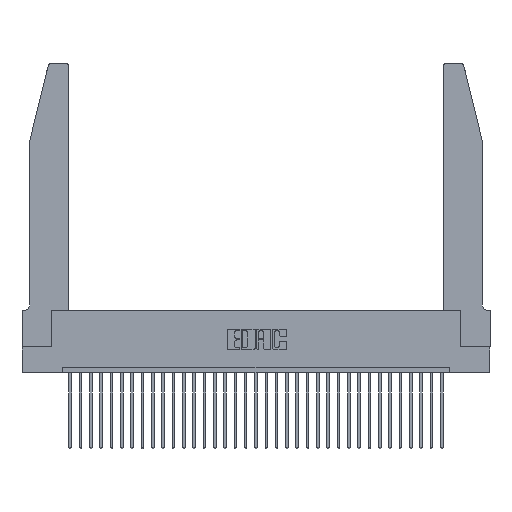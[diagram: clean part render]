
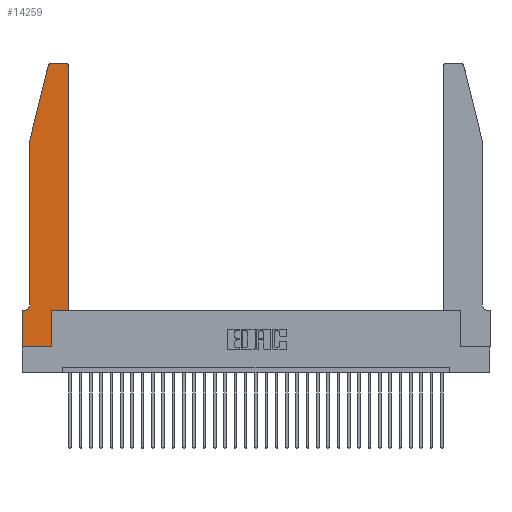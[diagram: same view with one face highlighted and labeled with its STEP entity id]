
A CAD part, top view. The second image highlights one B-rep face of the part: STEP entity #14259.
In plain terms, the highlighted planar face has unit normal (0, 0, 1).
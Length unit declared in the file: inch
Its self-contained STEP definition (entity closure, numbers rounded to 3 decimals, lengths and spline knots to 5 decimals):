
#778 = EDGE_CURVE ( 'NONE', #25420, #25887, #30744, .T. ) ;
#1574 = VERTEX_POINT ( 'NONE', #26260 ) ;
#1593 = PLANE ( 'NONE',  #13772 ) ;
#1702 = EDGE_CURVE ( 'NONE', #33284, #24533, #17965, .T. ) ;
#1807 = CARTESIAN_POINT ( 'NONE',  ( 0.0755, 2., 0.37 ) ) ;
#2394 = VECTOR ( 'NONE', #32917, 39.37008 ) ;
#2762 = CARTESIAN_POINT ( 'NONE',  ( 0.284, 2.75, 0.37 ) ) ;
#3095 = VERTEX_POINT ( 'NONE', #2762 ) ;
#3455 = FACE_OUTER_BOUND ( 'NONE', #14669, .T. ) ;
#3578 = EDGE_CURVE ( 'NONE', #28450, #33284, #10489, .T. ) ;
#3635 = VECTOR ( 'NONE', #14544, 39.37008 ) ;
#4038 = DIRECTION ( 'NONE',  ( 0., -1., 0. ) ) ;
#4308 = VECTOR ( 'NONE', #7700, 39.37008 ) ;
#4322 = ORIENTED_EDGE ( 'NONE', *, *, #15088, .T. ) ;
#4743 = EDGE_CURVE ( 'NONE', #12954, #25420, #31672, .T. ) ;
#4748 = EDGE_CURVE ( 'NONE', #25887, #8091, #14783, .T. ) ;
#4892 = EDGE_CURVE ( 'NONE', #21681, #3095, #24809, .T. ) ;
#4966 = ORIENTED_EDGE ( 'NONE', *, *, #29760, .T. ) ;
#5181 = DIRECTION ( 'NONE',  ( 1., 0., 0. ) ) ;
#5616 = VECTOR ( 'NONE', #30119, 39.37008 ) ;
#5626 = CARTESIAN_POINT ( 'NONE',  ( 0.4505, 2.72, 0.37 ) ) ;
#5845 = VECTOR ( 'NONE', #23015, 39.37008 ) ;
#7334 = CARTESIAN_POINT ( 'NONE',  ( 0., 0.35, 0.37 ) ) ;
#7700 = DIRECTION ( 'NONE',  ( 0., 1., 0. ) ) ;
#7824 = DIRECTION ( 'NONE',  ( -1., 0., 0. ) ) ;
#8091 = VERTEX_POINT ( 'NONE', #5626 ) ;
#9091 = CARTESIAN_POINT ( 'NONE',  ( 0.0755, 0.35, 0.37 ) ) ;
#9144 = AXIS2_PLACEMENT_3D ( 'NONE', #24869, #17339, #30339 ) ;
#10373 = VERTEX_POINT ( 'NONE', #7334 ) ;
#10489 = LINE ( 'NONE', #1807, #3635 ) ;
#11004 = LINE ( 'NONE', #9091, #19389 ) ;
#11280 = EDGE_CURVE ( 'NONE', #32089, #12954, #12478, .T. ) ;
#11499 = DIRECTION ( 'NONE',  ( -1., 0., 0. ) ) ;
#11637 = CARTESIAN_POINT ( 'NONE',  ( 0.0755, 0.42, 0.37 ) ) ;
#11727 = CARTESIAN_POINT ( 'NONE',  ( 0.25487, 2.72718, 0.37 ) ) ;
#11792 = CARTESIAN_POINT ( 'NONE',  ( 0.4505, 0.35, 0.37 ) ) ;
#12034 = EDGE_CURVE ( 'NONE', #8091, #21681, #23751, .T. ) ;
#12143 = ORIENTED_EDGE ( 'NONE', *, *, #17559, .T. ) ;
#12462 = CARTESIAN_POINT ( 'NONE',  ( 0.4205, 2.75, 0.37 ) ) ;
#12478 = LINE ( 'NONE', #24864, #5616 ) ;
#12834 = ORIENTED_EDGE ( 'NONE', *, *, #3578, .T. ) ;
#12954 = VERTEX_POINT ( 'NONE', #18596 ) ;
#13772 = AXIS2_PLACEMENT_3D ( 'NONE', #29914, #17126, #14550 ) ;
#13867 = ORIENTED_EDGE ( 'NONE', *, *, #22809, .T. ) ;
#14259 = ADVANCED_FACE ( 'NONE', ( #3455 ), #1593, .T. ) ;
#14544 = DIRECTION ( 'NONE',  ( -0.239, -0.971, 0. ) ) ;
#14550 = DIRECTION ( 'NONE',  ( 1., 0., 0. ) ) ;
#14669 = EDGE_LOOP ( 'NONE', ( #24459, #4322, #12834, #25105, #4966, #13867, #12143, #27820, #32342, #16875, #18695, #23669 ) ) ;
#14783 = LINE ( 'NONE', #11792, #4308 ) ;
#14976 = CARTESIAN_POINT ( 'NONE',  ( 0., 0., 0.37 ) ) ;
#15088 = EDGE_CURVE ( 'NONE', #3095, #28450, #27484, .T. ) ;
#15936 = VECTOR ( 'NONE', #4038, 39.37008 ) ;
#16875 = ORIENTED_EDGE ( 'NONE', *, *, #778, .T. ) ;
#17126 = DIRECTION ( 'NONE',  ( 0., 0., 1. ) ) ;
#17339 = DIRECTION ( 'NONE',  ( 0., 0., -1. ) ) ;
#17559 = EDGE_CURVE ( 'NONE', #10373, #32089, #21348, .T. ) ;
#17965 = LINE ( 'NONE', #24729, #15936 ) ;
#18028 = AXIS2_PLACEMENT_3D ( 'NONE', #31439, #18799, #28959 ) ;
#18596 = CARTESIAN_POINT ( 'NONE',  ( 0.2865, 0., 0.37 ) ) ;
#18695 = ORIENTED_EDGE ( 'NONE', *, *, #4748, .T. ) ;
#18754 = AXIS2_PLACEMENT_3D ( 'NONE', #32943, #22741, #5181 ) ;
#18799 = DIRECTION ( 'NONE',  ( 0., 0., 1. ) ) ;
#19231 = VECTOR ( 'NONE', #22199, 39.37008 ) ;
#19389 = VECTOR ( 'NONE', #11499, 39.37008 ) ;
#19649 = CARTESIAN_POINT ( 'NONE',  ( 0.2865, 0.35, 0.37 ) ) ;
#19975 = CARTESIAN_POINT ( 'NONE',  ( 0.0755, 2., 0.37 ) ) ;
#21348 = LINE ( 'NONE', #14976, #2394 ) ;
#21681 = VERTEX_POINT ( 'NONE', #12462 ) ;
#21879 = CARTESIAN_POINT ( 'NONE',  ( 0.2865, 0.35, 0.37 ) ) ;
#22199 = DIRECTION ( 'NONE',  ( 0., 1., 0. ) ) ;
#22741 = DIRECTION ( 'NONE',  ( 0., 0., 1. ) ) ;
#22802 = VECTOR ( 'NONE', #7824, 39.37008 ) ;
#22809 = EDGE_CURVE ( 'NONE', #1574, #10373, #11004, .T. ) ;
#23015 = DIRECTION ( 'NONE',  ( 1., 0., 0. ) ) ;
#23669 = ORIENTED_EDGE ( 'NONE', *, *, #12034, .T. ) ;
#23751 = CIRCLE ( 'NONE', #18028, 0.03 ) ;
#24459 = ORIENTED_EDGE ( 'NONE', *, *, #4892, .T. ) ;
#24533 = VERTEX_POINT ( 'NONE', #11637 ) ;
#24729 = CARTESIAN_POINT ( 'NONE',  ( 0.0755, 2., 0.37 ) ) ;
#24809 = LINE ( 'NONE', #25927, #22802 ) ;
#24864 = CARTESIAN_POINT ( 'NONE',  ( 0., 0., 0.37 ) ) ;
#24869 = CARTESIAN_POINT ( 'NONE',  ( 0.0055, 0.42, 0.37 ) ) ;
#25105 = ORIENTED_EDGE ( 'NONE', *, *, #1702, .T. ) ;
#25420 = VERTEX_POINT ( 'NONE', #21879 ) ;
#25887 = VERTEX_POINT ( 'NONE', #31603 ) ;
#25927 = CARTESIAN_POINT ( 'NONE',  ( 0.2605, 2.75, 0.37 ) ) ;
#26260 = CARTESIAN_POINT ( 'NONE',  ( 0.0055, 0.35, 0.37 ) ) ;
#27484 = CIRCLE ( 'NONE', #18754, 0.03 ) ;
#27820 = ORIENTED_EDGE ( 'NONE', *, *, #11280, .T. ) ;
#28450 = VERTEX_POINT ( 'NONE', #11727 ) ;
#28959 = DIRECTION ( 'NONE',  ( 1., 0., 0. ) ) ;
#29653 = CIRCLE ( 'NONE', #9144, 0.07 ) ;
#29760 = EDGE_CURVE ( 'NONE', #24533, #1574, #29653, .T. ) ;
#29914 = CARTESIAN_POINT ( 'NONE',  ( 0., 0.35, 0.37 ) ) ;
#30119 = DIRECTION ( 'NONE',  ( 1., 0., 0. ) ) ;
#30339 = DIRECTION ( 'NONE',  ( -1., 0., 0. ) ) ;
#30744 = LINE ( 'NONE', #30827, #5845 ) ;
#30827 = CARTESIAN_POINT ( 'NONE',  ( 0.4505, 0.35, 0.37 ) ) ;
#31439 = CARTESIAN_POINT ( 'NONE',  ( 0.4205, 2.72, 0.37 ) ) ;
#31603 = CARTESIAN_POINT ( 'NONE',  ( 0.4505, 0.35, 0.37 ) ) ;
#31672 = LINE ( 'NONE', #19649, #19231 ) ;
#32089 = VERTEX_POINT ( 'NONE', #32908 ) ;
#32342 = ORIENTED_EDGE ( 'NONE', *, *, #4743, .T. ) ;
#32908 = CARTESIAN_POINT ( 'NONE',  ( 0., 0., 0.37 ) ) ;
#32917 = DIRECTION ( 'NONE',  ( 0., -1., 0. ) ) ;
#32943 = CARTESIAN_POINT ( 'NONE',  ( 0.284, 2.72, 0.37 ) ) ;
#33284 = VERTEX_POINT ( 'NONE', #19975 ) ;
